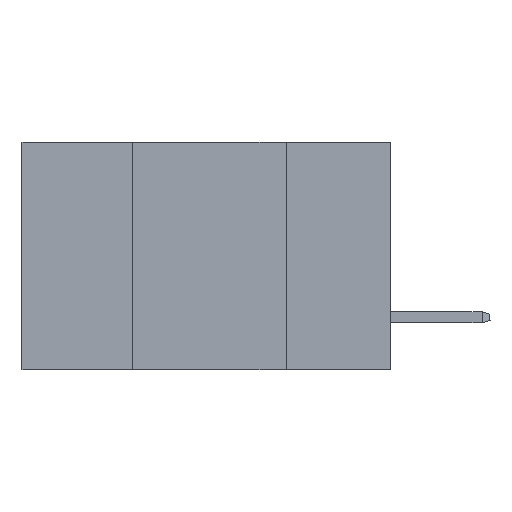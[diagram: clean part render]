
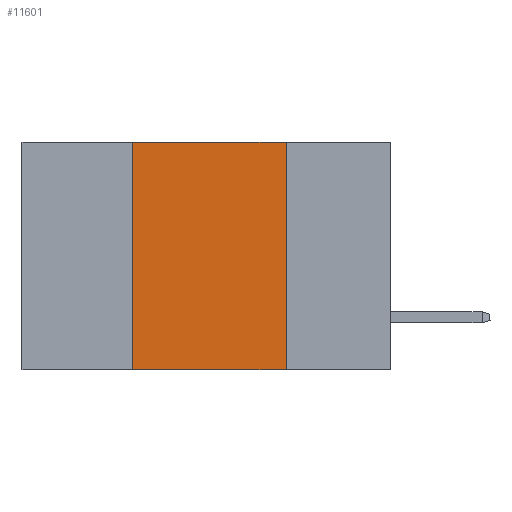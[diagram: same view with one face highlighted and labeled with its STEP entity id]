
A CAD part, left-side view. The second image highlights one B-rep face of the part: STEP entity #11601.
In plain terms, the highlighted planar face has unit normal (-1, 0, 0).
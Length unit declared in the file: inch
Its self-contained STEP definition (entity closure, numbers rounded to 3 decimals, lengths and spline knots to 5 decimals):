
#188 = ORIENTED_EDGE ( 'NONE', *, *, #1664, .F. ) ;
#887 = LINE ( 'NONE', #4443, #12370 ) ;
#1160 = DIRECTION ( 'NONE',  ( 0., 0., -1. ) ) ;
#1368 = EDGE_CURVE ( 'NONE', #3332, #2127, #8754, .T. ) ;
#1404 = PLANE ( 'NONE',  #11749 ) ;
#1664 = EDGE_CURVE ( 'NONE', #3332, #9477, #887, .T. ) ;
#2127 = VERTEX_POINT ( 'NONE', #4431 ) ;
#2303 = DIRECTION ( 'NONE',  ( 1., 0., 0. ) ) ;
#2677 = EDGE_LOOP ( 'NONE', ( #6771, #11522, #188, #7565 ) ) ;
#2699 = FACE_OUTER_BOUND ( 'NONE', #2677, .T. ) ;
#3069 = CARTESIAN_POINT ( 'NONE',  ( 0., 0.17, 0. ) ) ;
#3332 = VERTEX_POINT ( 'NONE', #4224 ) ;
#3747 = DIRECTION ( 'NONE',  ( 0., -1., 0. ) ) ;
#4030 = DIRECTION ( 'NONE',  ( 0., -1., 0. ) ) ;
#4224 = CARTESIAN_POINT ( 'NONE',  ( 0., 0.42, -0.37 ) ) ;
#4265 = DIRECTION ( 'NONE',  ( 0., 0., 1. ) ) ;
#4431 = CARTESIAN_POINT ( 'NONE',  ( 0., 0.17, -0.37 ) ) ;
#4443 = CARTESIAN_POINT ( 'NONE',  ( 0., 0.42, 0. ) ) ;
#4694 = LINE ( 'NONE', #3069, #7925 ) ;
#4921 = CARTESIAN_POINT ( 'NONE',  ( 0., 0.6, -0.37 ) ) ;
#6532 = EDGE_CURVE ( 'NONE', #7866, #2127, #4694, .T. ) ;
#6771 = ORIENTED_EDGE ( 'NONE', *, *, #6532, .F. ) ;
#6815 = CARTESIAN_POINT ( 'NONE',  ( 0., 0.6, 0. ) ) ;
#7214 = DIRECTION ( 'NONE',  ( 0., 0., -1. ) ) ;
#7565 = ORIENTED_EDGE ( 'NONE', *, *, #1368, .T. ) ;
#7866 = VERTEX_POINT ( 'NONE', #11642 ) ;
#7925 = VECTOR ( 'NONE', #1160, 39.37008 ) ;
#8424 = CARTESIAN_POINT ( 'NONE',  ( 0., 0.42, 0. ) ) ;
#8754 = LINE ( 'NONE', #4921, #11926 ) ;
#9477 = VERTEX_POINT ( 'NONE', #8424 ) ;
#9510 = LINE ( 'NONE', #6815, #10565 ) ;
#10565 = VECTOR ( 'NONE', #3747, 39.37008 ) ;
#10751 = EDGE_CURVE ( 'NONE', #9477, #7866, #9510, .T. ) ;
#11156 = CARTESIAN_POINT ( 'NONE',  ( 0., 0.6, 0. ) ) ;
#11522 = ORIENTED_EDGE ( 'NONE', *, *, #10751, .F. ) ;
#11601 = ADVANCED_FACE ( 'NONE', ( #2699 ), #1404, .F. ) ;
#11642 = CARTESIAN_POINT ( 'NONE',  ( 0., 0.17, 0. ) ) ;
#11749 = AXIS2_PLACEMENT_3D ( 'NONE', #11156, #2303, #7214 ) ;
#11926 = VECTOR ( 'NONE', #4030, 39.37008 ) ;
#12370 = VECTOR ( 'NONE', #4265, 39.37008 ) ;
